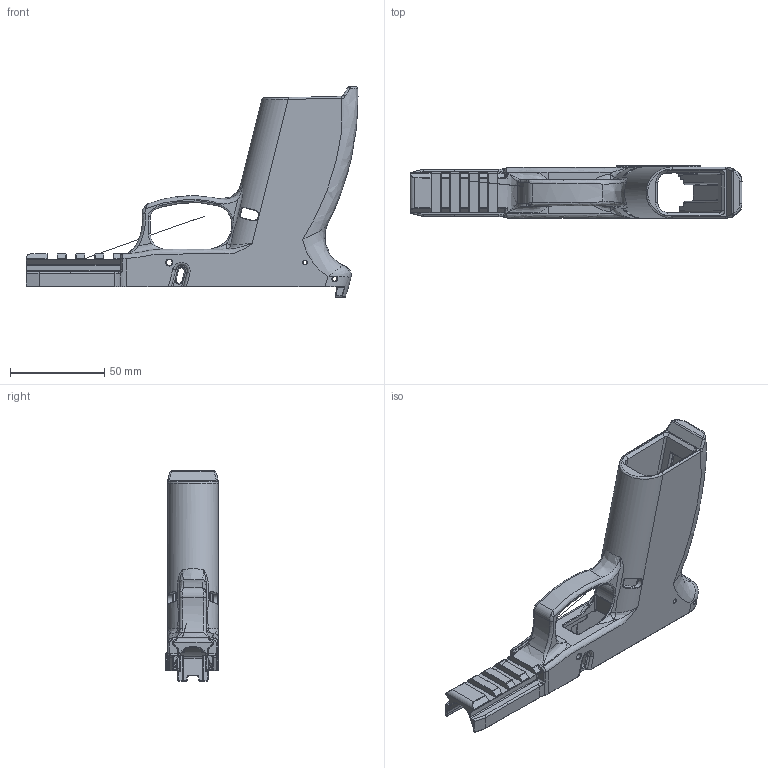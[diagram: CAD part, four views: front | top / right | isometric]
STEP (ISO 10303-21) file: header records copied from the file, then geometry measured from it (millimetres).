
FILE_DESCRIPTION(/* description */ (''),/* implementation_level */ '2;1');
FILE_NAME(/* name */ '//Wooly Bully - Taurus G3 Frame.step',/* time_stamp */ '2022-05-22T00:46:45-07:00',/* author */ (''),/* organization */ (''),/* preprocessor_version */ 'ST-DEVELOPER v18.1',/* originating_system */ 'Autodesk Translation Framework v10.14.0.1471',/* authorisation */ '');
FILE_SCHEMA (('AUTOMOTIVE_DESIGN { 1 0 10303 214 3 1 1 }'));
Products named in the file (1): (Unsaved)
Bounding box: 176.22 x 28 x 111.8 mm (x, y, z)
Volume: 84779.1 mm3; surface area: 42783.6 mm2
Topology: 1 solids, 1 shells, 1193 faces, 3408 edges, 2154 vertices
Faces by surface type: cylinder 475, bspline 283, plane 201, torus 195, cone 21, sphere 18
Full cylindrical faces by diameter (mm): 2 x2, 2.5 x2, 3.2 x2
Entity records: 230083 total; most frequent: CARTESIAN_POINT 200956, ORIENTED_EDGE 6708, DIRECTION 5477, EDGE_CURVE 3354, AXIS2_PLACEMENT_3D 2212, VERTEX_POINT 2154, EDGE_LOOP 1210, FACE_OUTER_BOUND 1193
